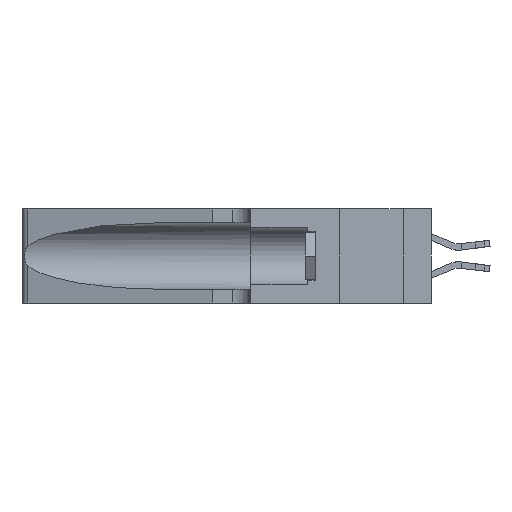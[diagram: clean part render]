
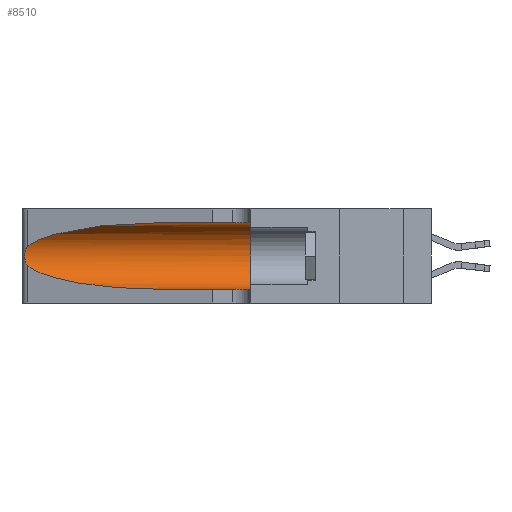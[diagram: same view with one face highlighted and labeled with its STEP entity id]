
A CAD part, left-side view. The second image highlights one B-rep face of the part: STEP entity #8510.
In plain terms, the highlighted cylindrical face has radius 3.308 mm (diameter 6.617 mm), a partial arc.
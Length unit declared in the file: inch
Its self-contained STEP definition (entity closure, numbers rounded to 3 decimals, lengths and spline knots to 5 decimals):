
#102 = ORIENTED_EDGE ( 'NONE', *, *, #23734, .T. ) ;
#128 = AXIS2_PLACEMENT_3D ( 'NONE', #3633, #16879, #1697 ) ;
#549 = CARTESIAN_POINT ( 'NONE',  ( 0.26075, 1.23896, 0.178 ) ) ;
#977 = EDGE_CURVE ( 'NONE', #11137, #1418, #2979, .T. ) ;
#1418 = VERTEX_POINT ( 'NONE', #13395 ) ;
#1697 = DIRECTION ( 'NONE',  ( 0., 0., -1. ) ) ;
#2476 = CARTESIAN_POINT ( 'NONE',  ( 0.25856, 1.23593, 0.16098 ) ) ;
#2521 = ORIENTED_EDGE ( 'NONE', *, *, #2738, .F. ) ;
#2538 = ORIENTED_EDGE ( 'NONE', *, *, #977, .T. ) ;
#2666 = B_SPLINE_CURVE_WITH_KNOTS ( 'NONE', 3,
 ( #21287, #19372, #8156, #21361, #10036, #23243, #11953, #549, #13861, #2476, #15756, #4419, #17648, #6320 ),
 .UNSPECIFIED., .F., .F.,
 ( 4, 2, 2, 2, 2, 2, 4 ),
 ( 0., 0.00027, 0.00053, 0.00107, 0.0016, 0.00187, 0.00214 ),
 .UNSPECIFIED. ) ;
#2738 = EDGE_CURVE ( 'NONE', #23284, #19492, #15317, .T. ) ;
#2979 =( BOUNDED_CURVE ( )  B_SPLINE_CURVE ( 3, ( #5250, #3853, #3080, #5233 ),
 .UNSPECIFIED., .F., .F. ) 
 B_SPLINE_CURVE_WITH_KNOTS ( ( 4, 4 ),
 ( 3.44316, 4.71239 ),
 .UNSPECIFIED. ) 
 CURVE ( )  GEOMETRIC_REPRESENTATION_ITEM ( )  RATIONAL_B_SPLINE_CURVE ( ( 1., 0.87, 0.87, 1. ) ) 
 REPRESENTATION_ITEM ( '' )  );
#3080 = CARTESIAN_POINT ( 'NONE',  ( 0.18966, 0.96281, 0.05475 ) ) ;
#3633 = CARTESIAN_POINT ( 'NONE',  ( 0.1305, 1.61858, 0.185 ) ) ;
#3853 = CARTESIAN_POINT ( 'NONE',  ( 0.2373, 1.15595, 0.08982 ) ) ;
#3998 = CYLINDRICAL_SURFACE ( 'NONE', #128, 0.13025 ) ;
#4163 = EDGE_CURVE ( 'NONE', #5395, #11137, #2666, .T. ) ;
#4419 = CARTESIAN_POINT ( 'NONE',  ( 0.25639, 1.23186, 0.15144 ) ) ;
#4578 = FACE_OUTER_BOUND ( 'NONE', #18895, .T. ) ;
#5233 = CARTESIAN_POINT ( 'NONE',  ( 0.1305, 0.72297, 0.05475 ) ) ;
#5250 = CARTESIAN_POINT ( 'NONE',  ( 0.25487, 1.22718, 0.14631 ) ) ;
#5395 = VERTEX_POINT ( 'NONE', #10726 ) ;
#5676 = CARTESIAN_POINT ( 'NONE',  ( 0.1305, 0.35, 0.05475 ) ) ;
#6098 = CIRCLE ( 'NONE', #21713, 0.13025 ) ;
#6231 = VERTEX_POINT ( 'NONE', #5676 ) ;
#6320 = CARTESIAN_POINT ( 'NONE',  ( 0.25487, 1.22718, 0.14631 ) ) ;
#7978 = CARTESIAN_POINT ( 'NONE',  ( 0.1305, 1.61858, 0.31525 ) ) ;
#8156 = CARTESIAN_POINT ( 'NONE',  ( 0.25639, 1.23184, 0.21858 ) ) ;
#8510 = ADVANCED_FACE ( 'NONE', ( #4578 ), #3998, .F. ) ;
#8846 = DIRECTION ( 'NONE',  ( 0., 1., 0. ) ) ;
#8882 = EDGE_CURVE ( 'NONE', #19492, #6231, #6098, .T. ) ;
#10036 = CARTESIAN_POINT ( 'NONE',  ( 0.25854, 1.2359, 0.20912 ) ) ;
#10271 = DIRECTION ( 'NONE',  ( 0., -1., 0. ) ) ;
#10726 = CARTESIAN_POINT ( 'NONE',  ( 0.25487, 1.22718, 0.22369 ) ) ;
#11137 = VERTEX_POINT ( 'NONE', #14273 ) ;
#11953 = CARTESIAN_POINT ( 'NONE',  ( 0.26075, 1.23896, 0.19203 ) ) ;
#12253 =( BOUNDED_CURVE ( )  B_SPLINE_CURVE ( 3, ( #20500, #18601, #24297, #13012 ),
 .UNSPECIFIED., .F., .F. ) 
 B_SPLINE_CURVE_WITH_KNOTS ( ( 4, 4 ),
 ( 1.5708, 2.84003 ),
 .UNSPECIFIED. ) 
 CURVE ( )  GEOMETRIC_REPRESENTATION_ITEM ( )  RATIONAL_B_SPLINE_CURVE ( ( 1., 0.87, 0.87, 1. ) ) 
 REPRESENTATION_ITEM ( '' )  );
#13012 = CARTESIAN_POINT ( 'NONE',  ( 0.25487, 1.22718, 0.22369 ) ) ;
#13395 = CARTESIAN_POINT ( 'NONE',  ( 0.1305, 0.72297, 0.05475 ) ) ;
#13640 = ORIENTED_EDGE ( 'NONE', *, *, #8882, .F. ) ;
#13861 = CARTESIAN_POINT ( 'NONE',  ( 0.26017, 1.23833, 0.17102 ) ) ;
#14273 = CARTESIAN_POINT ( 'NONE',  ( 0.25487, 1.22718, 0.14631 ) ) ;
#15317 = LINE ( 'NONE', #7978, #19711 ) ;
#15372 = ORIENTED_EDGE ( 'NONE', *, *, #15749, .T. ) ;
#15749 = EDGE_CURVE ( 'NONE', #1418, #6231, #22410, .T. ) ;
#15756 = CARTESIAN_POINT ( 'NONE',  ( 0.25789, 1.23486, 0.15765 ) ) ;
#16879 = DIRECTION ( 'NONE',  ( 0., -1., 0. ) ) ;
#17405 = CARTESIAN_POINT ( 'NONE',  ( 0.1305, 0.72297, 0.31525 ) ) ;
#17648 = CARTESIAN_POINT ( 'NONE',  ( 0.25555, 1.22993, 0.14849 ) ) ;
#18601 = CARTESIAN_POINT ( 'NONE',  ( 0.18966, 0.96281, 0.31525 ) ) ;
#18895 = EDGE_LOOP ( 'NONE', ( #102, #19972, #2538, #15372, #13640, #2521 ) ) ;
#19372 = CARTESIAN_POINT ( 'NONE',  ( 0.25555, 1.22994, 0.2215 ) ) ;
#19492 = VERTEX_POINT ( 'NONE', #20614 ) ;
#19711 = VECTOR ( 'NONE', #23074, 39.37008 ) ;
#19972 = ORIENTED_EDGE ( 'NONE', *, *, #4163, .T. ) ;
#20148 = CARTESIAN_POINT ( 'NONE',  ( 0.1305, 0.35, 0.185 ) ) ;
#20500 = CARTESIAN_POINT ( 'NONE',  ( 0.1305, 0.72297, 0.31525 ) ) ;
#20614 = CARTESIAN_POINT ( 'NONE',  ( 0.1305, 0.35, 0.31525 ) ) ;
#21287 = CARTESIAN_POINT ( 'NONE',  ( 0.25487, 1.22718, 0.22369 ) ) ;
#21361 = CARTESIAN_POINT ( 'NONE',  ( 0.25787, 1.23484, 0.2124 ) ) ;
#21713 = AXIS2_PLACEMENT_3D ( 'NONE', #20148, #8846, #22046 ) ;
#21814 = VECTOR ( 'NONE', #10271, 39.37008 ) ;
#22046 = DIRECTION ( 'NONE',  ( 0., 0., 1. ) ) ;
#22410 = LINE ( 'NONE', #23473, #21814 ) ;
#23074 = DIRECTION ( 'NONE',  ( 0., -1., 0. ) ) ;
#23243 = CARTESIAN_POINT ( 'NONE',  ( 0.26018, 1.23835, 0.19895 ) ) ;
#23284 = VERTEX_POINT ( 'NONE', #17405 ) ;
#23473 = CARTESIAN_POINT ( 'NONE',  ( 0.1305, 1.61858, 0.05475 ) ) ;
#23734 = EDGE_CURVE ( 'NONE', #23284, #5395, #12253, .T. ) ;
#24297 = CARTESIAN_POINT ( 'NONE',  ( 0.2373, 1.15595, 0.28018 ) ) ;
